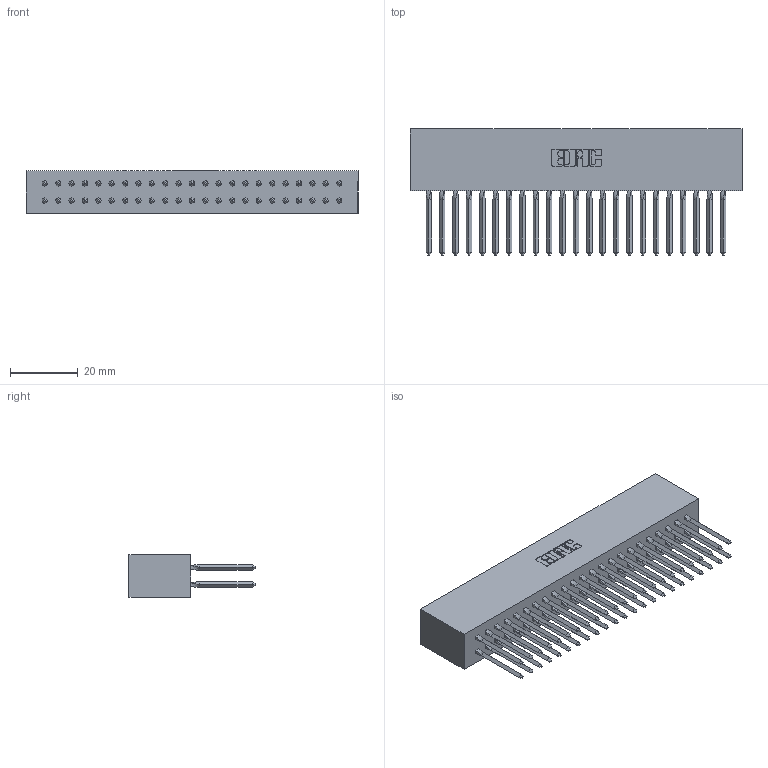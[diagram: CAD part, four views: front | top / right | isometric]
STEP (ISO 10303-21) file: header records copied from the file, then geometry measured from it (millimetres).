
FILE_DESCRIPTION (( 'STEP AP203' ), '1' );
FILE_NAME ('317-046-542-801.STEP', '2020-02-28T02:25:02', ( '' ), ( '' ), 'SwSTEP 2.0', 'SolidWorks 2016', '' );
FILE_SCHEMA (( 'CONFIG_CONTROL_DESIGN' ));
Length unit declared in the file: inch
Products named in the file (3): 317-046-542-801; 317-290-003_542; 317 Part_Lugless
Assembly tree (47 placements, depth 2):
  317-046-542-801
    317 Part_Lugless
    317-290-003_542  x46
Bounding box: 98.35 x 37.34 x 12.7 mm (x, y, z)
Volume: 17234.1 mm3; surface area: 23532.7 mm2
Topology: 47 solids, 47 shells, 2712 faces, 7599 edges, 4850 vertices
Faces by surface type: plane 2166, cylinder 362, bspline 184
Entity records: 34505 total; most frequent: CARTESIAN_POINT 6265, ORIENTED_EDGE 5928, DIRECTION 5012, EDGE_CURVE 2964, VECTOR 2802, LINE 2802, VERTEX_POINT 1970, AXIS2_PLACEMENT_3D 1105
